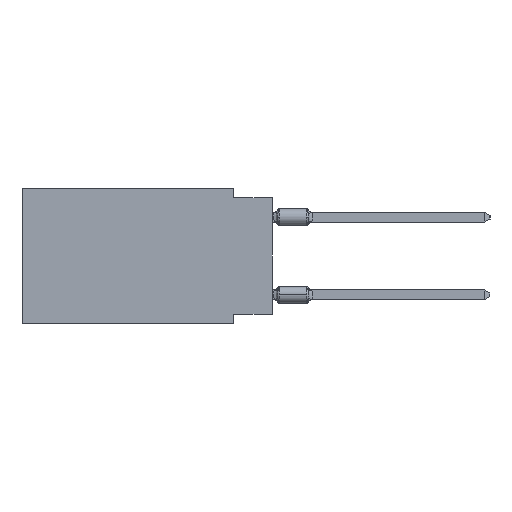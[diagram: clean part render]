
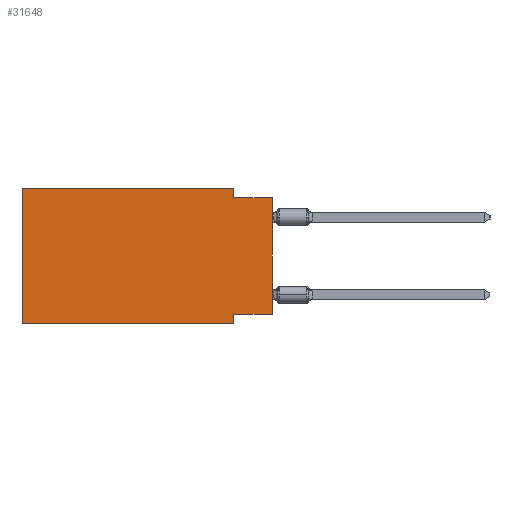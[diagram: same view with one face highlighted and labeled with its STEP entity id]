
A CAD part, left-side view. The second image highlights one B-rep face of the part: STEP entity #31648.
In plain terms, the highlighted planar face has unit normal (-1, 0, 0).
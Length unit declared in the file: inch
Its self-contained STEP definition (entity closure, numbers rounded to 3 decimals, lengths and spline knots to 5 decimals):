
#193 = VECTOR ( 'NONE', #21435, 39.37008 ) ;
#425 = EDGE_CURVE ( 'NONE', #7113, #16411, #32224, .T. ) ;
#1217 = VERTEX_POINT ( 'NONE', #16623 ) ;
#1593 = CARTESIAN_POINT ( 'NONE',  ( 0., 0.645, 0. ) ) ;
#2212 = CARTESIAN_POINT ( 'NONE',  ( 0., 0.645, -0.35 ) ) ;
#2801 = CARTESIAN_POINT ( 'NONE',  ( 0., 0., 0. ) ) ;
#3259 = LINE ( 'NONE', #6745, #30487 ) ;
#3855 = DIRECTION ( 'NONE',  ( 0., -1., 0. ) ) ;
#3873 = ORIENTED_EDGE ( 'NONE', *, *, #40407, .F. ) ;
#3980 = EDGE_CURVE ( 'NONE', #8154, #16411, #13241, .T. ) ;
#4624 = CARTESIAN_POINT ( 'NONE',  ( 0., 0.1, -0.325 ) ) ;
#4711 = FACE_OUTER_BOUND ( 'NONE', #9214, .T. ) ;
#5297 = CARTESIAN_POINT ( 'NONE',  ( 0., 0.1, -0.35 ) ) ;
#5319 = DIRECTION ( 'NONE',  ( 1., 0., 0. ) ) ;
#6106 = EDGE_CURVE ( 'NONE', #7502, #7113, #6831, .T. ) ;
#6745 = CARTESIAN_POINT ( 'NONE',  ( 0., 0.1, 0. ) ) ;
#6831 = LINE ( 'NONE', #25864, #25399 ) ;
#7113 = VERTEX_POINT ( 'NONE', #4624 ) ;
#7502 = VERTEX_POINT ( 'NONE', #12211 ) ;
#7531 = VERTEX_POINT ( 'NONE', #40441 ) ;
#7678 = CARTESIAN_POINT ( 'NONE',  ( 0., 0.1, -0.35 ) ) ;
#8154 = VERTEX_POINT ( 'NONE', #2212 ) ;
#8232 = VECTOR ( 'NONE', #19790, 39.37008 ) ;
#9214 = EDGE_LOOP ( 'NONE', ( #14382, #24051, #3873, #9645, #34853, #29646, #34580, #28724 ) ) ;
#9645 = ORIENTED_EDGE ( 'NONE', *, *, #29366, .F. ) ;
#11183 = VECTOR ( 'NONE', #3855, 39.37008 ) ;
#11837 = LINE ( 'NONE', #2801, #12636 ) ;
#12211 = CARTESIAN_POINT ( 'NONE',  ( 0., 0., -0.325 ) ) ;
#12630 = VECTOR ( 'NONE', #39914, 39.37008 ) ;
#12636 = VECTOR ( 'NONE', #24315, 39.37008 ) ;
#12757 = CARTESIAN_POINT ( 'NONE',  ( 0., 0.645, 0. ) ) ;
#13241 = LINE ( 'NONE', #25913, #8232 ) ;
#13597 = CARTESIAN_POINT ( 'NONE',  ( 0., 0., -0.025 ) ) ;
#14382 = ORIENTED_EDGE ( 'NONE', *, *, #34860, .T. ) ;
#14954 = VERTEX_POINT ( 'NONE', #12757 ) ;
#16411 = VERTEX_POINT ( 'NONE', #5297 ) ;
#16623 = CARTESIAN_POINT ( 'NONE',  ( 0., 0.1, -0.025 ) ) ;
#17040 = PLANE ( 'NONE',  #21007 ) ;
#17947 = CARTESIAN_POINT ( 'NONE',  ( 0., 0., -0.025 ) ) ;
#18052 = CARTESIAN_POINT ( 'NONE',  ( 0., 0.645, 0. ) ) ;
#18971 = VECTOR ( 'NONE', #25903, 39.37008 ) ;
#19790 = DIRECTION ( 'NONE',  ( 0., -1., 0. ) ) ;
#21007 = AXIS2_PLACEMENT_3D ( 'NONE', #29497, #5319, #29902 ) ;
#21435 = DIRECTION ( 'NONE',  ( 0., -1., 0. ) ) ;
#21878 = VERTEX_POINT ( 'NONE', #13597 ) ;
#24051 = ORIENTED_EDGE ( 'NONE', *, *, #35367, .F. ) ;
#24315 = DIRECTION ( 'NONE',  ( 0., 0., 1. ) ) ;
#25399 = VECTOR ( 'NONE', #34883, 39.37008 ) ;
#25864 = CARTESIAN_POINT ( 'NONE',  ( 0., 0., -0.325 ) ) ;
#25903 = DIRECTION ( 'NONE',  ( 0., 0., -1. ) ) ;
#25913 = CARTESIAN_POINT ( 'NONE',  ( 0., 0.645, -0.35 ) ) ;
#27086 = EDGE_CURVE ( 'NONE', #8154, #14954, #27444, .T. ) ;
#27444 = LINE ( 'NONE', #18052, #12630 ) ;
#28724 = ORIENTED_EDGE ( 'NONE', *, *, #6106, .F. ) ;
#28847 = LINE ( 'NONE', #1593, #11183 ) ;
#29366 = EDGE_CURVE ( 'NONE', #14954, #7531, #28847, .T. ) ;
#29497 = CARTESIAN_POINT ( 'NONE',  ( 0., 0.645, 0. ) ) ;
#29646 = ORIENTED_EDGE ( 'NONE', *, *, #3980, .T. ) ;
#29902 = DIRECTION ( 'NONE',  ( 0., 0., -1. ) ) ;
#30487 = VECTOR ( 'NONE', #35197, 39.37008 ) ;
#31648 = ADVANCED_FACE ( 'NONE', ( #4711 ), #17040, .F. ) ;
#32224 = LINE ( 'NONE', #7678, #18971 ) ;
#34580 = ORIENTED_EDGE ( 'NONE', *, *, #425, .F. ) ;
#34853 = ORIENTED_EDGE ( 'NONE', *, *, #27086, .F. ) ;
#34860 = EDGE_CURVE ( 'NONE', #7502, #21878, #11837, .T. ) ;
#34883 = DIRECTION ( 'NONE',  ( 0., 1., 0. ) ) ;
#35197 = DIRECTION ( 'NONE',  ( 0., 0., -1. ) ) ;
#35367 = EDGE_CURVE ( 'NONE', #1217, #21878, #39814, .T. ) ;
#39814 = LINE ( 'NONE', #17947, #193 ) ;
#39914 = DIRECTION ( 'NONE',  ( 0., 0., 1. ) ) ;
#40407 = EDGE_CURVE ( 'NONE', #7531, #1217, #3259, .T. ) ;
#40441 = CARTESIAN_POINT ( 'NONE',  ( 0., 0.1, 0. ) ) ;
